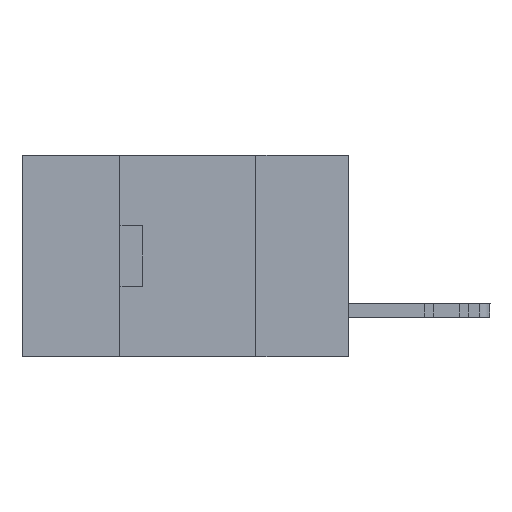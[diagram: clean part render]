
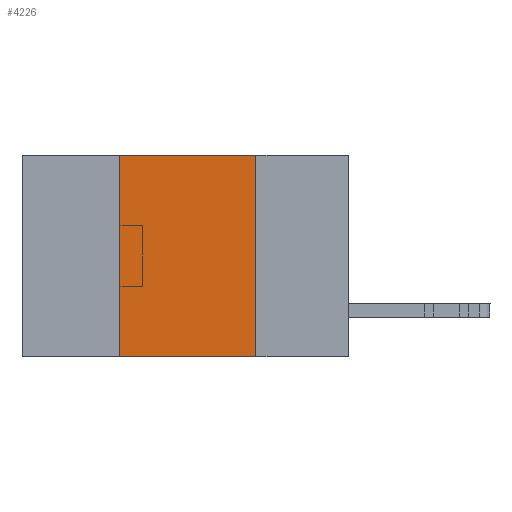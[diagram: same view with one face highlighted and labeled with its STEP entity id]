
A CAD part, left-side view. The second image highlights one B-rep face of the part: STEP entity #4226.
In plain terms, the highlighted planar face has unit normal (-1, 0, 0).
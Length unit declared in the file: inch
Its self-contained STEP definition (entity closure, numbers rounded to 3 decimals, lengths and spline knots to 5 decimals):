
#1893 = VERTEX_POINT ( 'NONE', #17677 ) ;
#1957 = ORIENTED_EDGE ( 'NONE', *, *, #17902, .T. ) ;
#3769 = EDGE_CURVE ( 'NONE', #24467, #26236, #9854, .T. ) ;
#4058 = DIRECTION ( 'NONE',  ( 0., 0., 1. ) ) ;
#4226 = ADVANCED_FACE ( 'NONE', ( #17888 ), #7942, .F. ) ;
#4923 = LINE ( 'NONE', #11487, #6979 ) ;
#5491 = ORIENTED_EDGE ( 'NONE', *, *, #3769, .F. ) ;
#6022 = VERTEX_POINT ( 'NONE', #15264 ) ;
#6085 = DIRECTION ( 'NONE',  ( 0., 0., -1. ) ) ;
#6304 = EDGE_LOOP ( 'NONE', ( #5491, #15241, #23243, #1957 ) ) ;
#6721 = EDGE_CURVE ( 'NONE', #6022, #1893, #14238, .T. ) ;
#6979 = VECTOR ( 'NONE', #17544, 39.37008 ) ;
#7942 = PLANE ( 'NONE',  #14736 ) ;
#9854 = LINE ( 'NONE', #14137, #22863 ) ;
#11487 = CARTESIAN_POINT ( 'NONE',  ( 0., 0.6, 0. ) ) ;
#11709 = CARTESIAN_POINT ( 'NONE',  ( 0., 0.17, 0. ) ) ;
#12658 = DIRECTION ( 'NONE',  ( 0., -1., 0. ) ) ;
#13450 = VECTOR ( 'NONE', #12658, 39.37008 ) ;
#14137 = CARTESIAN_POINT ( 'NONE',  ( 0., 0.17, -0.37 ) ) ;
#14238 = LINE ( 'NONE', #22425, #20412 ) ;
#14736 = AXIS2_PLACEMENT_3D ( 'NONE', #16122, #26164, #16256 ) ;
#15241 = ORIENTED_EDGE ( 'NONE', *, *, #15565, .F. ) ;
#15264 = CARTESIAN_POINT ( 'NONE',  ( 0., 0.42, -0.37 ) ) ;
#15565 = EDGE_CURVE ( 'NONE', #1893, #24467, #4923, .T. ) ;
#16122 = CARTESIAN_POINT ( 'NONE',  ( 0., 0.6, 0. ) ) ;
#16256 = DIRECTION ( 'NONE',  ( 0., 0., -1. ) ) ;
#17544 = DIRECTION ( 'NONE',  ( 0., -1., 0. ) ) ;
#17677 = CARTESIAN_POINT ( 'NONE',  ( 0., 0.42, 0. ) ) ;
#17822 = CARTESIAN_POINT ( 'NONE',  ( 0., 0.17, -0.37 ) ) ;
#17888 = FACE_OUTER_BOUND ( 'NONE', #6304, .T. ) ;
#17902 = EDGE_CURVE ( 'NONE', #6022, #26236, #19103, .T. ) ;
#18590 = CARTESIAN_POINT ( 'NONE',  ( 0., 0.6, -0.37 ) ) ;
#19103 = LINE ( 'NONE', #18590, #13450 ) ;
#20412 = VECTOR ( 'NONE', #4058, 39.37008 ) ;
#22425 = CARTESIAN_POINT ( 'NONE',  ( 0., 0.42, -0.37 ) ) ;
#22863 = VECTOR ( 'NONE', #6085, 39.37008 ) ;
#23243 = ORIENTED_EDGE ( 'NONE', *, *, #6721, .F. ) ;
#24467 = VERTEX_POINT ( 'NONE', #11709 ) ;
#26164 = DIRECTION ( 'NONE',  ( 1., 0., 0. ) ) ;
#26236 = VERTEX_POINT ( 'NONE', #17822 ) ;
